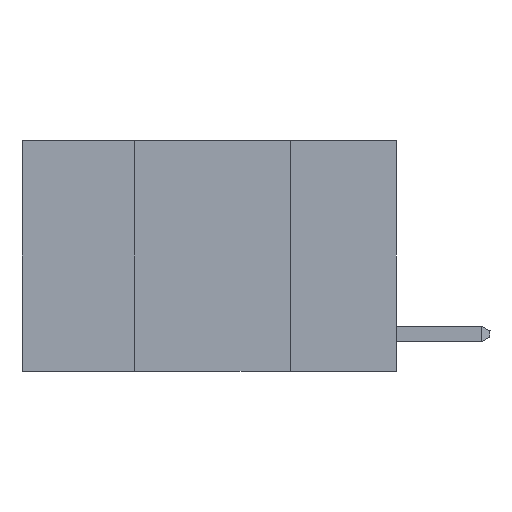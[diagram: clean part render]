
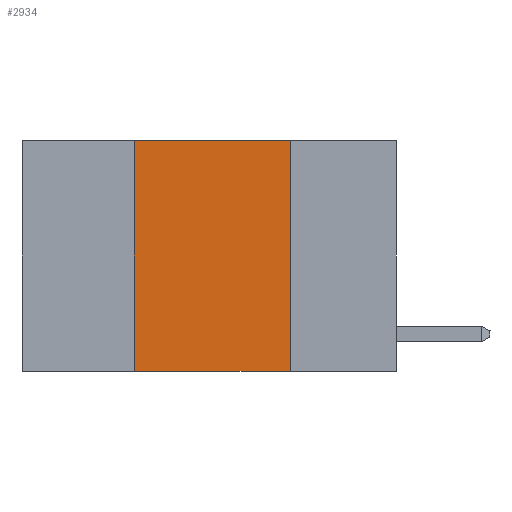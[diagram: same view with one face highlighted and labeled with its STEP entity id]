
A CAD part, left-side view. The second image highlights one B-rep face of the part: STEP entity #2934.
In plain terms, the highlighted planar face has unit normal (-1, 0, 0).
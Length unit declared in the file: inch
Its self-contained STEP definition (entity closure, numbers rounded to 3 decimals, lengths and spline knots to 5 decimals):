
#51 = CARTESIAN_POINT ( 'NONE',  ( 0., 0.17, 0. ) ) ;
#278 = LINE ( 'NONE', #17059, #8082 ) ;
#1000 = ORIENTED_EDGE ( 'NONE', *, *, #7981, .F. ) ;
#1321 = AXIS2_PLACEMENT_3D ( 'NONE', #7467, #17788, #2316 ) ;
#1937 = EDGE_CURVE ( 'NONE', #12136, #13215, #278, .T. ) ;
#2316 = DIRECTION ( 'NONE',  ( 0., 0., -1. ) ) ;
#2908 = CARTESIAN_POINT ( 'NONE',  ( 0., 0.6, 0. ) ) ;
#2934 = ADVANCED_FACE ( 'NONE', ( #12516 ), #14275, .F. ) ;
#3035 = LINE ( 'NONE', #51, #13007 ) ;
#3106 = EDGE_LOOP ( 'NONE', ( #12227, #6209, #1000, #14862 ) ) ;
#3122 = DIRECTION ( 'NONE',  ( 0., -1., 0. ) ) ;
#3889 = VECTOR ( 'NONE', #15848, 39.37008 ) ;
#4093 = VERTEX_POINT ( 'NONE', #6108 ) ;
#4600 = CARTESIAN_POINT ( 'NONE',  ( 0., 0.42, 0. ) ) ;
#5279 = CARTESIAN_POINT ( 'NONE',  ( 0., 0.42, -0.37 ) ) ;
#6108 = CARTESIAN_POINT ( 'NONE',  ( 0., 0.17, 0. ) ) ;
#6209 = ORIENTED_EDGE ( 'NONE', *, *, #10023, .F. ) ;
#6677 = VECTOR ( 'NONE', #16668, 39.37008 ) ;
#6912 = EDGE_CURVE ( 'NONE', #4093, #13215, #3035, .T. ) ;
#7074 = DIRECTION ( 'NONE',  ( 0., 0., -1. ) ) ;
#7467 = CARTESIAN_POINT ( 'NONE',  ( 0., 0.6, 0. ) ) ;
#7975 = LINE ( 'NONE', #2908, #6677 ) ;
#7981 = EDGE_CURVE ( 'NONE', #12136, #9156, #9721, .T. ) ;
#8082 = VECTOR ( 'NONE', #3122, 39.37008 ) ;
#8299 = CARTESIAN_POINT ( 'NONE',  ( 0., 0.17, -0.37 ) ) ;
#9156 = VERTEX_POINT ( 'NONE', #11794 ) ;
#9721 = LINE ( 'NONE', #4600, #3889 ) ;
#10023 = EDGE_CURVE ( 'NONE', #9156, #4093, #7975, .T. ) ;
#11794 = CARTESIAN_POINT ( 'NONE',  ( 0., 0.42, 0. ) ) ;
#12136 = VERTEX_POINT ( 'NONE', #5279 ) ;
#12227 = ORIENTED_EDGE ( 'NONE', *, *, #6912, .F. ) ;
#12516 = FACE_OUTER_BOUND ( 'NONE', #3106, .T. ) ;
#13007 = VECTOR ( 'NONE', #7074, 39.37008 ) ;
#13215 = VERTEX_POINT ( 'NONE', #8299 ) ;
#14275 = PLANE ( 'NONE',  #1321 ) ;
#14862 = ORIENTED_EDGE ( 'NONE', *, *, #1937, .T. ) ;
#15848 = DIRECTION ( 'NONE',  ( 0., 0., 1. ) ) ;
#16668 = DIRECTION ( 'NONE',  ( 0., -1., 0. ) ) ;
#17059 = CARTESIAN_POINT ( 'NONE',  ( 0., 0.6, -0.37 ) ) ;
#17788 = DIRECTION ( 'NONE',  ( 1., 0., 0. ) ) ;
